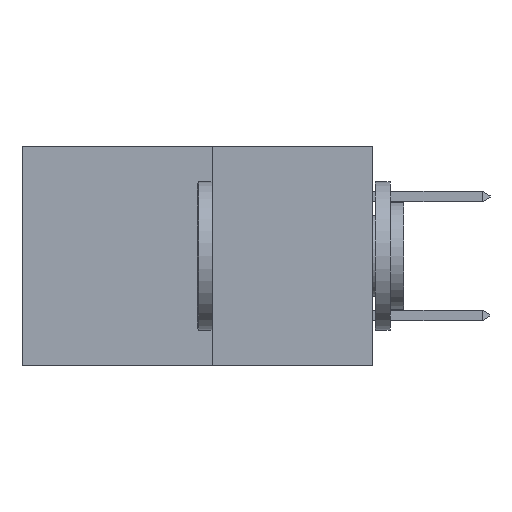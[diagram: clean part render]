
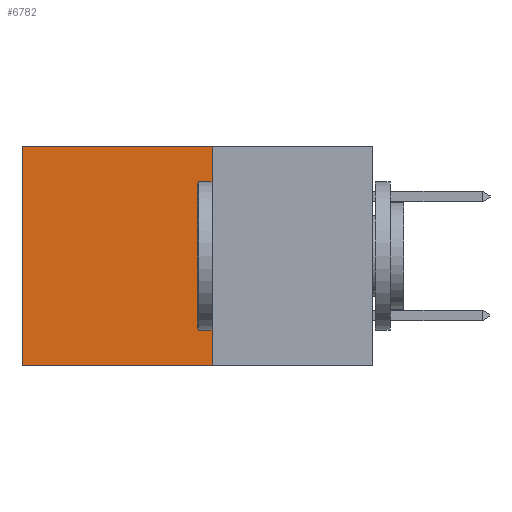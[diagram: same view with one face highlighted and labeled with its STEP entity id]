
A CAD part, left-side view. The second image highlights one B-rep face of the part: STEP entity #6782.
In plain terms, the highlighted planar face has unit normal (-1, 0, 0).
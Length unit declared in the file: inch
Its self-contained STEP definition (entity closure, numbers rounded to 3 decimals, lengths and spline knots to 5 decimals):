
#167 = CARTESIAN_POINT ( 'NONE',  ( 0.277, 0.59, 0. ) ) ;
#243 = VERTEX_POINT ( 'NONE', #4424 ) ;
#864 = ORIENTED_EDGE ( 'NONE', *, *, #1277, .T. ) ;
#980 = LINE ( 'NONE', #8008, #4403 ) ;
#1043 = FACE_OUTER_BOUND ( 'NONE', #3349, .T. ) ;
#1236 = PLANE ( 'NONE',  #7476 ) ;
#1263 = LINE ( 'NONE', #7391, #4429 ) ;
#1277 = EDGE_CURVE ( 'NONE', #2937, #5629, #1263, .T. ) ;
#1372 = CARTESIAN_POINT ( 'NONE',  ( 0.277, 0.27, 0. ) ) ;
#1587 = DIRECTION ( 'NONE',  ( 0., 0., -1. ) ) ;
#1860 = LINE ( 'NONE', #4936, #3601 ) ;
#1992 = DIRECTION ( 'NONE',  ( 0., 0., -1. ) ) ;
#2002 = EDGE_CURVE ( 'NONE', #4089, #243, #5914, .T. ) ;
#2119 = DIRECTION ( 'NONE',  ( 1., 0., 0. ) ) ;
#2243 = CARTESIAN_POINT ( 'NONE',  ( 0.277, 0.27, -0.37 ) ) ;
#2937 = VERTEX_POINT ( 'NONE', #167 ) ;
#3080 = EDGE_CURVE ( 'NONE', #4089, #2937, #1860, .T. ) ;
#3349 = EDGE_LOOP ( 'NONE', ( #864, #8358, #4560, #8776 ) ) ;
#3601 = VECTOR ( 'NONE', #8745, 39.37008 ) ;
#3642 = DIRECTION ( 'NONE',  ( 0., 0., -1. ) ) ;
#3940 = EDGE_CURVE ( 'NONE', #243, #5629, #980, .T. ) ;
#4089 = VERTEX_POINT ( 'NONE', #1372 ) ;
#4403 = VECTOR ( 'NONE', #6900, 39.37008 ) ;
#4424 = CARTESIAN_POINT ( 'NONE',  ( 0.277, 0.27, -0.37 ) ) ;
#4429 = VECTOR ( 'NONE', #3642, 39.37008 ) ;
#4560 = ORIENTED_EDGE ( 'NONE', *, *, #2002, .F. ) ;
#4936 = CARTESIAN_POINT ( 'NONE',  ( 0.277, 0.27, 0. ) ) ;
#5473 = CARTESIAN_POINT ( 'NONE',  ( 0.277, 0.27, -0.37 ) ) ;
#5629 = VERTEX_POINT ( 'NONE', #8188 ) ;
#5914 = LINE ( 'NONE', #5473, #7857 ) ;
#6782 = ADVANCED_FACE ( 'NONE', ( #1043 ), #1236, .F. ) ;
#6900 = DIRECTION ( 'NONE',  ( 0., 1., 0. ) ) ;
#7391 = CARTESIAN_POINT ( 'NONE',  ( 0.277, 0.59, -0.37 ) ) ;
#7476 = AXIS2_PLACEMENT_3D ( 'NONE', #2243, #2119, #1992 ) ;
#7857 = VECTOR ( 'NONE', #1587, 39.37008 ) ;
#8008 = CARTESIAN_POINT ( 'NONE',  ( 0.277, 0.27, -0.37 ) ) ;
#8188 = CARTESIAN_POINT ( 'NONE',  ( 0.277, 0.59, -0.37 ) ) ;
#8358 = ORIENTED_EDGE ( 'NONE', *, *, #3940, .F. ) ;
#8745 = DIRECTION ( 'NONE',  ( 0., 1., 0. ) ) ;
#8776 = ORIENTED_EDGE ( 'NONE', *, *, #3080, .T. ) ;
